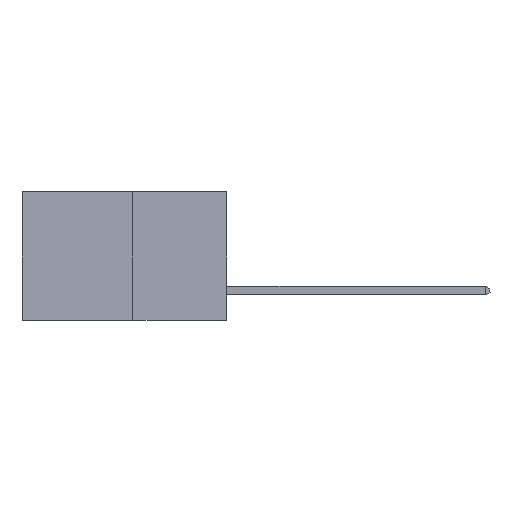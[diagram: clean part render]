
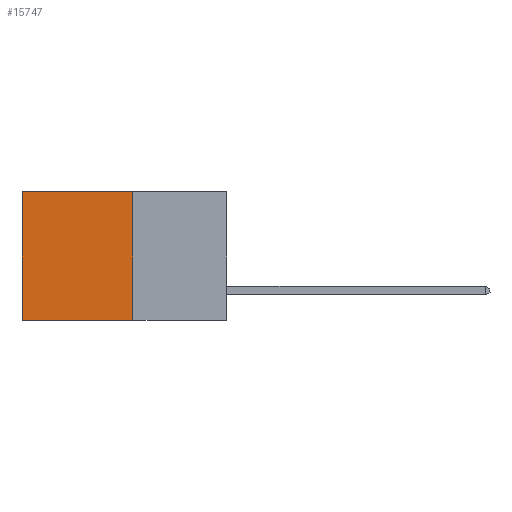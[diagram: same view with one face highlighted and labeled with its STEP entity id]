
A CAD part, left-side view. The second image highlights one B-rep face of the part: STEP entity #15747.
In plain terms, the highlighted planar face has unit normal (-1, 0, 0).
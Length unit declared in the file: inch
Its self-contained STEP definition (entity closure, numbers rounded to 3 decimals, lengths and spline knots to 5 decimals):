
#577 = VECTOR ( 'NONE', #13858, 39.37008 ) ;
#2181 = CARTESIAN_POINT ( 'NONE',  ( 0.277, 0.27, 0. ) ) ;
#2281 = CARTESIAN_POINT ( 'NONE',  ( 0.277, 0.27, -0.37 ) ) ;
#2599 = VECTOR ( 'NONE', #11360, 39.37008 ) ;
#3036 = VECTOR ( 'NONE', #3471, 39.37008 ) ;
#3471 = DIRECTION ( 'NONE',  ( 0., 1., 0. ) ) ;
#4380 = LINE ( 'NONE', #13394, #577 ) ;
#6110 = PLANE ( 'NONE',  #6873 ) ;
#6292 = VERTEX_POINT ( 'NONE', #12316 ) ;
#6700 = EDGE_CURVE ( 'NONE', #15023, #14616, #4380, .T. ) ;
#6873 = AXIS2_PLACEMENT_3D ( 'NONE', #2281, #7394, #15960 ) ;
#7193 = ORIENTED_EDGE ( 'NONE', *, *, #14952, .T. ) ;
#7394 = DIRECTION ( 'NONE',  ( 1., 0., 0. ) ) ;
#7727 = ORIENTED_EDGE ( 'NONE', *, *, #6700, .F. ) ;
#7791 = ORIENTED_EDGE ( 'NONE', *, *, #15230, .F. ) ;
#8512 = ORIENTED_EDGE ( 'NONE', *, *, #13256, .T. ) ;
#8628 = EDGE_LOOP ( 'NONE', ( #7193, #7727, #7791, #8512 ) ) ;
#8707 = CARTESIAN_POINT ( 'NONE',  ( 0.277, 0.59, 0. ) ) ;
#9752 = LINE ( 'NONE', #2181, #3036 ) ;
#10165 = CARTESIAN_POINT ( 'NONE',  ( 0.277, 0.27, -0.37 ) ) ;
#10186 = CARTESIAN_POINT ( 'NONE',  ( 0.277, 0.59, -0.37 ) ) ;
#10805 = DIRECTION ( 'NONE',  ( 0., 0., -1. ) ) ;
#10998 = FACE_OUTER_BOUND ( 'NONE', #8628, .T. ) ;
#11360 = DIRECTION ( 'NONE',  ( 0., 0., -1. ) ) ;
#12154 = LINE ( 'NONE', #10165, #2599 ) ;
#12316 = CARTESIAN_POINT ( 'NONE',  ( 0.277, 0.27, 0. ) ) ;
#13132 = VECTOR ( 'NONE', #10805, 39.37008 ) ;
#13247 = CARTESIAN_POINT ( 'NONE',  ( 0.277, 0.59, -0.37 ) ) ;
#13256 = EDGE_CURVE ( 'NONE', #6292, #15120, #9752, .T. ) ;
#13394 = CARTESIAN_POINT ( 'NONE',  ( 0.277, 0.27, -0.37 ) ) ;
#13506 = LINE ( 'NONE', #13247, #13132 ) ;
#13858 = DIRECTION ( 'NONE',  ( 0., 1., 0. ) ) ;
#14576 = CARTESIAN_POINT ( 'NONE',  ( 0.277, 0.27, -0.37 ) ) ;
#14616 = VERTEX_POINT ( 'NONE', #10186 ) ;
#14952 = EDGE_CURVE ( 'NONE', #15120, #14616, #13506, .T. ) ;
#15023 = VERTEX_POINT ( 'NONE', #14576 ) ;
#15120 = VERTEX_POINT ( 'NONE', #8707 ) ;
#15230 = EDGE_CURVE ( 'NONE', #6292, #15023, #12154, .T. ) ;
#15747 = ADVANCED_FACE ( 'NONE', ( #10998 ), #6110, .F. ) ;
#15960 = DIRECTION ( 'NONE',  ( 0., 0., -1. ) ) ;
